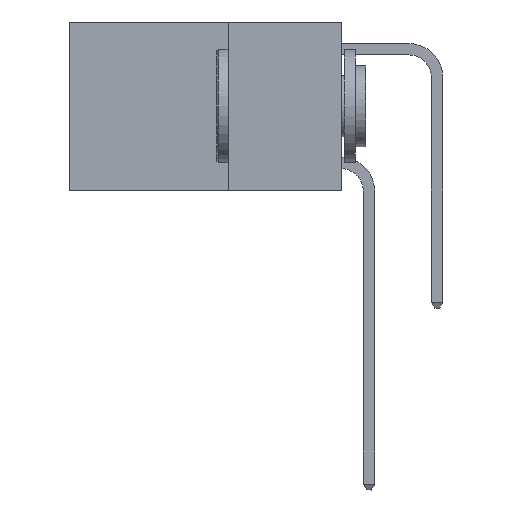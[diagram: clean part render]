
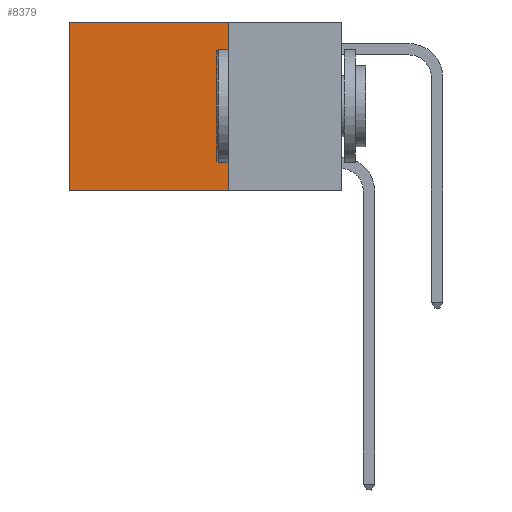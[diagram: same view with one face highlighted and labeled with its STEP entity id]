
A CAD part, left-side view. The second image highlights one B-rep face of the part: STEP entity #8379.
In plain terms, the highlighted planar face has unit normal (-1, 0, 0).
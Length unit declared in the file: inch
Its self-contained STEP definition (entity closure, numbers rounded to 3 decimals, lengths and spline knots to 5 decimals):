
#165 = CARTESIAN_POINT ( 'NONE',  ( 0.2625, 0.25, -0.37 ) ) ;
#1076 = VERTEX_POINT ( 'NONE', #6243 ) ;
#1213 = ORIENTED_EDGE ( 'NONE', *, *, #7258, .T. ) ;
#1706 = CARTESIAN_POINT ( 'NONE',  ( 0.2625, 0.6, 0. ) ) ;
#1825 = CARTESIAN_POINT ( 'NONE',  ( 0.2625, 0.6, -0.37 ) ) ;
#2098 = EDGE_LOOP ( 'NONE', ( #12516, #9187, #10276, #1213 ) ) ;
#2630 = DIRECTION ( 'NONE',  ( 0., 1., 0. ) ) ;
#3059 = VERTEX_POINT ( 'NONE', #8486 ) ;
#3914 = FACE_OUTER_BOUND ( 'NONE', #2098, .T. ) ;
#3947 = DIRECTION ( 'NONE',  ( 0., 0., -1. ) ) ;
#4629 = EDGE_CURVE ( 'NONE', #3059, #13769, #5968, .T. ) ;
#5169 = VERTEX_POINT ( 'NONE', #10536 ) ;
#5267 = EDGE_CURVE ( 'NONE', #5169, #13769, #6988, .T. ) ;
#5770 = VECTOR ( 'NONE', #10583, 39.37008 ) ;
#5784 = DIRECTION ( 'NONE',  ( 0., 1., 0. ) ) ;
#5968 = LINE ( 'NONE', #165, #14081 ) ;
#6241 = VECTOR ( 'NONE', #2630, 39.37008 ) ;
#6243 = CARTESIAN_POINT ( 'NONE',  ( 0.2625, 0.25, 0. ) ) ;
#6913 = LINE ( 'NONE', #9618, #13299 ) ;
#6988 = LINE ( 'NONE', #1706, #5770 ) ;
#7126 = PLANE ( 'NONE',  #8063 ) ;
#7258 = EDGE_CURVE ( 'NONE', #1076, #5169, #11780, .T. ) ;
#7675 = EDGE_CURVE ( 'NONE', #1076, #3059, #6913, .T. ) ;
#8063 = AXIS2_PLACEMENT_3D ( 'NONE', #9453, #10575, #3947 ) ;
#8379 = ADVANCED_FACE ( 'NONE', ( #3914 ), #7126, .F. ) ;
#8486 = CARTESIAN_POINT ( 'NONE',  ( 0.2625, 0.25, -0.37 ) ) ;
#9187 = ORIENTED_EDGE ( 'NONE', *, *, #4629, .F. ) ;
#9336 = CARTESIAN_POINT ( 'NONE',  ( 0.2625, 0.25, 0. ) ) ;
#9453 = CARTESIAN_POINT ( 'NONE',  ( 0.2625, 0.25, 0. ) ) ;
#9618 = CARTESIAN_POINT ( 'NONE',  ( 0.2625, 0.25, 0. ) ) ;
#10276 = ORIENTED_EDGE ( 'NONE', *, *, #7675, .F. ) ;
#10536 = CARTESIAN_POINT ( 'NONE',  ( 0.2625, 0.6, 0. ) ) ;
#10575 = DIRECTION ( 'NONE',  ( 1., 0., 0. ) ) ;
#10583 = DIRECTION ( 'NONE',  ( 0., 0., -1. ) ) ;
#11274 = DIRECTION ( 'NONE',  ( 0., 0., -1. ) ) ;
#11780 = LINE ( 'NONE', #9336, #6241 ) ;
#12516 = ORIENTED_EDGE ( 'NONE', *, *, #5267, .T. ) ;
#13299 = VECTOR ( 'NONE', #11274, 39.37008 ) ;
#13769 = VERTEX_POINT ( 'NONE', #1825 ) ;
#14081 = VECTOR ( 'NONE', #5784, 39.37008 ) ;
